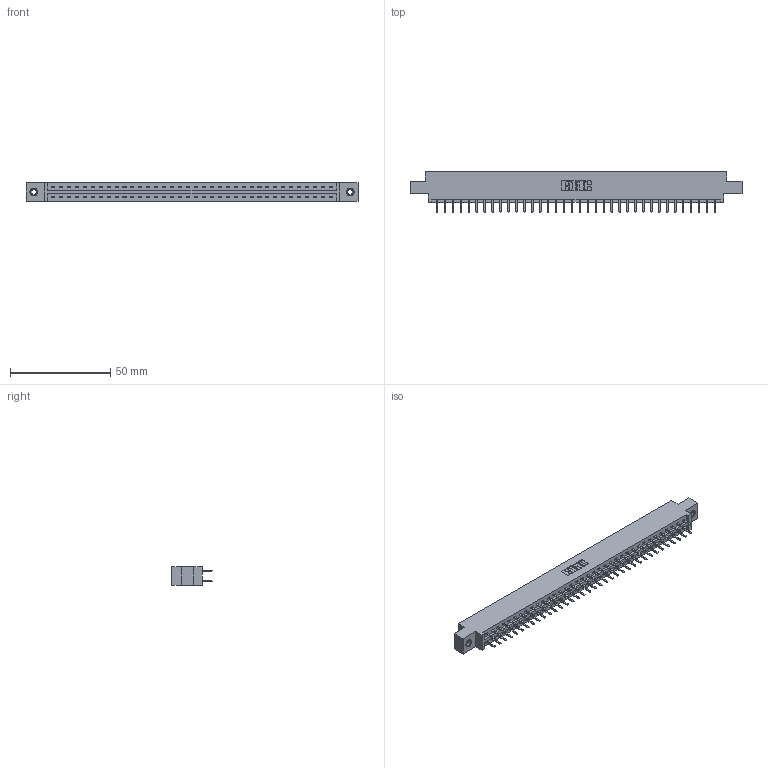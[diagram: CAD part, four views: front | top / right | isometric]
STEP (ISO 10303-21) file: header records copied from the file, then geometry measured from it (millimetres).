
FILE_DESCRIPTION (( 'STEP AP203' ), '1' );
FILE_NAME ('337-072-520-808.STEP', '2018-08-11T13:57:57', ( '' ), ( '' ), 'SwSTEP 2.0', 'SolidWorks 2016', '' );
FILE_SCHEMA (( 'CONFIG_CONTROL_DESIGN' ));
Length unit declared in the file: inch
Products named in the file (4): 337 Part_0.170 Offset - 0.156 Dia-TI; 345-292-001_345-293-120; 345-250-001_345-250-003-102; 337-072-520-808
Assembly tree (75 placements, depth 2):
  337-072-520-808
    337 Part_0.170 Offset - 0.156 Dia-TI
    345-292-001_345-293-120  x72
    345-250-001_345-250-003-102  x2
Bounding box: 165.66 x 20.02 x 9.4 mm (x, y, z)
Volume: 17222.9 mm3; surface area: 19453.7 mm2
Topology: 75 solids, 75 shells, 4354 faces, 12627 edges, 8218 vertices
Faces by surface type: plane 2986, cylinder 1352, cone 12, torus 4
Entity records: 30120 total; most frequent: CARTESIAN_POINT 5073, ORIENTED_EDGE 4990, DIRECTION 4345, EDGE_CURVE 2495, LINE 2343, VECTOR 2343, VERTEX_POINT 1656, AXIS2_PLACEMENT_3D 1001
